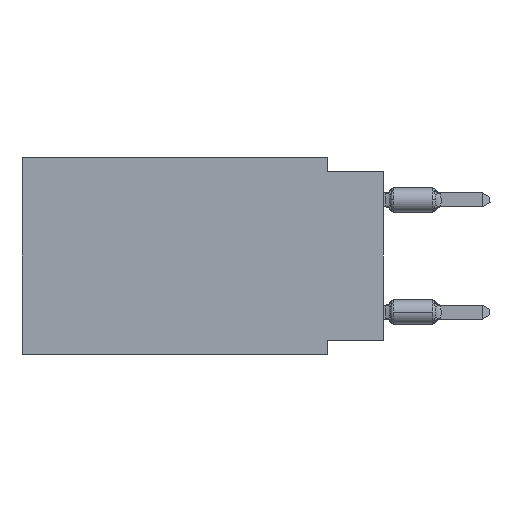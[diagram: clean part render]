
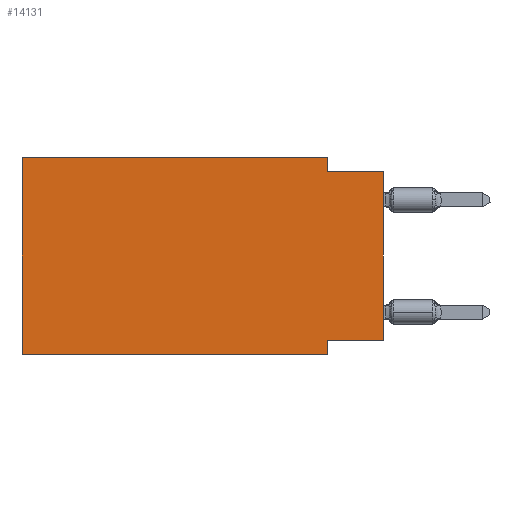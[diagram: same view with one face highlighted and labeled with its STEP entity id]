
A CAD part, left-side view. The second image highlights one B-rep face of the part: STEP entity #14131.
In plain terms, the highlighted planar face has unit normal (-1, 0, 0).
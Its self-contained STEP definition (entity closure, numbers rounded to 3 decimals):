
#359 = LINE ( 'NONE', #21243, #18010 ) ;
#493 = CARTESIAN_POINT ( 'NONE',  ( 0., 16.383, 0. ) ) ;
#762 = ORIENTED_EDGE ( 'NONE', *, *, #5766, .F. ) ;
#1109 = DIRECTION ( 'NONE',  ( 0., 0., 1. ) ) ;
#1355 = VECTOR ( 'NONE', #1109, 1000. ) ;
#2585 = EDGE_CURVE ( 'NONE', #26644, #7213, #14416, .T. ) ;
#2855 = LINE ( 'NONE', #493, #28287 ) ;
#3001 = CARTESIAN_POINT ( 'NONE',  ( 0., 0., -8.255 ) ) ;
#3393 = LINE ( 'NONE', #22520, #18978 ) ;
#3791 = CARTESIAN_POINT ( 'NONE',  ( 0., 0., 0. ) ) ;
#4249 = PLANE ( 'NONE',  #16287 ) ;
#4602 = CARTESIAN_POINT ( 'NONE',  ( 0., 16.383, -8.89 ) ) ;
#4770 = DIRECTION ( 'NONE',  ( 0., 0., -1. ) ) ;
#5263 = CARTESIAN_POINT ( 'NONE',  ( 0., 2.54, -8.255 ) ) ;
#5433 = ORIENTED_EDGE ( 'NONE', *, *, #2585, .F. ) ;
#5639 = EDGE_LOOP ( 'NONE', ( #13937, #762, #5433, #18400, #25656, #8771, #11222, #26409 ) ) ;
#5766 = EDGE_CURVE ( 'NONE', #7213, #25555, #3393, .T. ) ;
#6133 = VECTOR ( 'NONE', #24000, 1000. ) ;
#6637 = EDGE_CURVE ( 'NONE', #30737, #25555, #18208, .T. ) ;
#6855 = DIRECTION ( 'NONE',  ( 0., -1., 0. ) ) ;
#7213 = VERTEX_POINT ( 'NONE', #12144 ) ;
#7302 = LINE ( 'NONE', #11865, #7379 ) ;
#7379 = VECTOR ( 'NONE', #6855, 1000. ) ;
#7607 = CARTESIAN_POINT ( 'NONE',  ( 0., 16.383, 0. ) ) ;
#7672 = VERTEX_POINT ( 'NONE', #4602 ) ;
#7822 = VECTOR ( 'NONE', #17250, 1000. ) ;
#8771 = ORIENTED_EDGE ( 'NONE', *, *, #15552, .T. ) ;
#8789 = CARTESIAN_POINT ( 'NONE',  ( 0., 0., -8.255 ) ) ;
#10376 = VERTEX_POINT ( 'NONE', #5263 ) ;
#10675 = VERTEX_POINT ( 'NONE', #13865 ) ;
#11222 = ORIENTED_EDGE ( 'NONE', *, *, #30290, .F. ) ;
#11865 = CARTESIAN_POINT ( 'NONE',  ( 0., 16.383, 0. ) ) ;
#12144 = CARTESIAN_POINT ( 'NONE',  ( 0., 2.54, -0.635 ) ) ;
#12535 = LINE ( 'NONE', #26977, #7822 ) ;
#13865 = CARTESIAN_POINT ( 'NONE',  ( 0., 2.54, -8.89 ) ) ;
#13914 = EDGE_CURVE ( 'NONE', #7672, #23171, #2855, .T. ) ;
#13937 = ORIENTED_EDGE ( 'NONE', *, *, #6637, .T. ) ;
#14131 = ADVANCED_FACE ( 'NONE', ( #28245 ), #4249, .F. ) ;
#14416 = LINE ( 'NONE', #14568, #6133 ) ;
#14568 = CARTESIAN_POINT ( 'NONE',  ( 0., 2.54, 0. ) ) ;
#15552 = EDGE_CURVE ( 'NONE', #7672, #10675, #12535, .T. ) ;
#15621 = DIRECTION ( 'NONE',  ( 0., -1., 0. ) ) ;
#16156 = DIRECTION ( 'NONE',  ( 0., 1., 0. ) ) ;
#16287 = AXIS2_PLACEMENT_3D ( 'NONE', #16938, #21177, #23539 ) ;
#16938 = CARTESIAN_POINT ( 'NONE',  ( 0., 16.383, 0. ) ) ;
#17250 = DIRECTION ( 'NONE',  ( 0., -1., 0. ) ) ;
#17760 = CARTESIAN_POINT ( 'NONE',  ( 0., 2.54, 0. ) ) ;
#18010 = VECTOR ( 'NONE', #4770, 1000. ) ;
#18208 = LINE ( 'NONE', #3791, #1355 ) ;
#18400 = ORIENTED_EDGE ( 'NONE', *, *, #25070, .F. ) ;
#18978 = VECTOR ( 'NONE', #15621, 1000. ) ;
#20230 = LINE ( 'NONE', #8789, #23513 ) ;
#21177 = DIRECTION ( 'NONE',  ( 1., 0., 0. ) ) ;
#21243 = CARTESIAN_POINT ( 'NONE',  ( 0., 2.54, -8.89 ) ) ;
#22520 = CARTESIAN_POINT ( 'NONE',  ( 0., 0., -0.635 ) ) ;
#23171 = VERTEX_POINT ( 'NONE', #7607 ) ;
#23513 = VECTOR ( 'NONE', #16156, 1000. ) ;
#23539 = DIRECTION ( 'NONE',  ( 0., 0., -1. ) ) ;
#24000 = DIRECTION ( 'NONE',  ( 0., 0., -1. ) ) ;
#25070 = EDGE_CURVE ( 'NONE', #23171, #26644, #7302, .T. ) ;
#25555 = VERTEX_POINT ( 'NONE', #29519 ) ;
#25656 = ORIENTED_EDGE ( 'NONE', *, *, #13914, .F. ) ;
#26409 = ORIENTED_EDGE ( 'NONE', *, *, #28618, .F. ) ;
#26644 = VERTEX_POINT ( 'NONE', #17760 ) ;
#26977 = CARTESIAN_POINT ( 'NONE',  ( 0., 16.383, -8.89 ) ) ;
#28245 = FACE_OUTER_BOUND ( 'NONE', #5639, .T. ) ;
#28287 = VECTOR ( 'NONE', #29656, 1000. ) ;
#28618 = EDGE_CURVE ( 'NONE', #30737, #10376, #20230, .T. ) ;
#29519 = CARTESIAN_POINT ( 'NONE',  ( 0., 0., -0.635 ) ) ;
#29656 = DIRECTION ( 'NONE',  ( 0., 0., 1. ) ) ;
#30290 = EDGE_CURVE ( 'NONE', #10376, #10675, #359, .T. ) ;
#30737 = VERTEX_POINT ( 'NONE', #3001 ) ;
